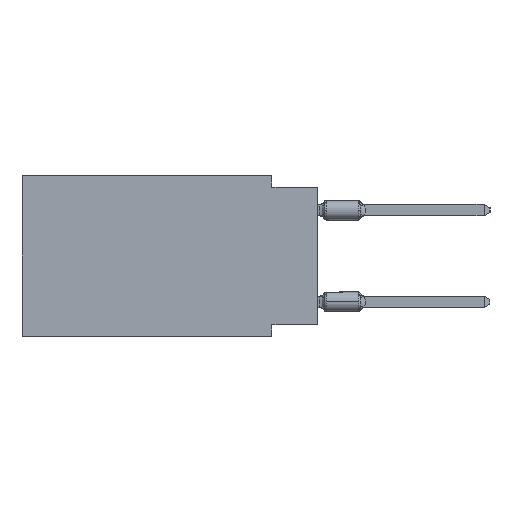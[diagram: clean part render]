
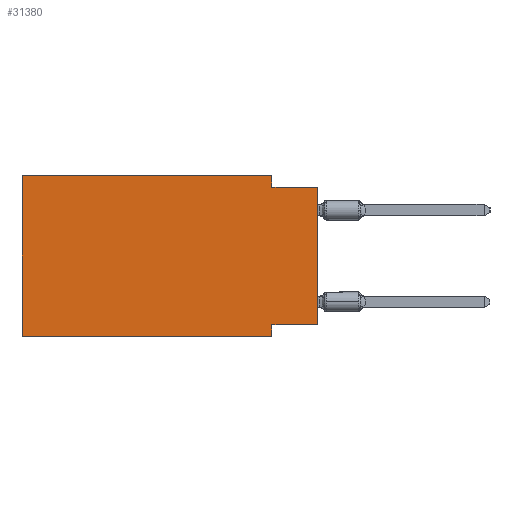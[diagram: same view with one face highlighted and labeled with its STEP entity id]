
A CAD part, left-side view. The second image highlights one B-rep face of the part: STEP entity #31380.
In plain terms, the highlighted planar face has unit normal (-1, 0, 0).
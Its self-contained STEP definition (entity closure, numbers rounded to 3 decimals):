
#2015 = EDGE_CURVE ( 'NONE', #42631, #43121, #25389, .T. ) ;
#2794 = DIRECTION ( 'NONE',  ( 0., 0., 1. ) ) ;
#2954 = VECTOR ( 'NONE', #29183, 1000. ) ;
#3737 = AXIS2_PLACEMENT_3D ( 'NONE', #24663, #42346, #38806 ) ;
#4232 = LINE ( 'NONE', #17900, #43510 ) ;
#5500 = FACE_OUTER_BOUND ( 'NONE', #38453, .T. ) ;
#5886 = ORIENTED_EDGE ( 'NONE', *, *, #20736, .F. ) ;
#5915 = CARTESIAN_POINT ( 'NONE',  ( 0., 16.383, -8.89 ) ) ;
#6879 = DIRECTION ( 'NONE',  ( 0., 0., 1. ) ) ;
#7085 = DIRECTION ( 'NONE',  ( 0., -1., 0. ) ) ;
#9016 = CARTESIAN_POINT ( 'NONE',  ( 0., 16.383, -8.89 ) ) ;
#10177 = EDGE_CURVE ( 'NONE', #32610, #34046, #17028, .T. ) ;
#10207 = CARTESIAN_POINT ( 'NONE',  ( 0., 2.54, -0.635 ) ) ;
#11324 = EDGE_CURVE ( 'NONE', #40060, #34046, #4232, .T. ) ;
#15069 = VECTOR ( 'NONE', #2794, 1000. ) ;
#16110 = EDGE_CURVE ( 'NONE', #40060, #19717, #24995, .T. ) ;
#16838 = ORIENTED_EDGE ( 'NONE', *, *, #10177, .F. ) ;
#17028 = LINE ( 'NONE', #37306, #37783 ) ;
#17112 = CARTESIAN_POINT ( 'NONE',  ( 0., 0., -0.635 ) ) ;
#17409 = VECTOR ( 'NONE', #41638, 1000. ) ;
#17900 = CARTESIAN_POINT ( 'NONE',  ( 0., 0., 0. ) ) ;
#18295 = CARTESIAN_POINT ( 'NONE',  ( 0., 0., -8.255 ) ) ;
#18673 = CARTESIAN_POINT ( 'NONE',  ( 0., 2.54, -8.89 ) ) ;
#18843 = CARTESIAN_POINT ( 'NONE',  ( 0., 0., -8.255 ) ) ;
#19096 = LINE ( 'NONE', #25693, #40429 ) ;
#19513 = EDGE_CURVE ( 'NONE', #33516, #29248, #35731, .T. ) ;
#19717 = VERTEX_POINT ( 'NONE', #30192 ) ;
#19989 = CARTESIAN_POINT ( 'NONE',  ( 0., 16.383, 0. ) ) ;
#20736 = EDGE_CURVE ( 'NONE', #19717, #29248, #19096, .T. ) ;
#20992 = VECTOR ( 'NONE', #22105, 1000. ) ;
#21790 = CARTESIAN_POINT ( 'NONE',  ( 0., 2.54, 0. ) ) ;
#22040 = ORIENTED_EDGE ( 'NONE', *, *, #2015, .F. ) ;
#22105 = DIRECTION ( 'NONE',  ( 0., -1., 0. ) ) ;
#23414 = ORIENTED_EDGE ( 'NONE', *, *, #41847, .F. ) ;
#24663 = CARTESIAN_POINT ( 'NONE',  ( 0., 16.383, 0. ) ) ;
#24995 = LINE ( 'NONE', #18843, #2954 ) ;
#25018 = ORIENTED_EDGE ( 'NONE', *, *, #39048, .F. ) ;
#25321 = DIRECTION ( 'NONE',  ( 0., -1., 0. ) ) ;
#25389 = LINE ( 'NONE', #35139, #20992 ) ;
#25693 = CARTESIAN_POINT ( 'NONE',  ( 0., 2.54, -8.89 ) ) ;
#26971 = ORIENTED_EDGE ( 'NONE', *, *, #11324, .T. ) ;
#29183 = DIRECTION ( 'NONE',  ( 0., 1., 0. ) ) ;
#29248 = VERTEX_POINT ( 'NONE', #18673 ) ;
#30192 = CARTESIAN_POINT ( 'NONE',  ( 0., 2.54, -8.255 ) ) ;
#31380 = ADVANCED_FACE ( 'NONE', ( #5500 ), #31759, .F. ) ;
#31759 = PLANE ( 'NONE',  #3737 ) ;
#32483 = ORIENTED_EDGE ( 'NONE', *, *, #16110, .F. ) ;
#32610 = VERTEX_POINT ( 'NONE', #10207 ) ;
#32993 = DIRECTION ( 'NONE',  ( 0., 0., -1. ) ) ;
#33516 = VERTEX_POINT ( 'NONE', #5915 ) ;
#34046 = VERTEX_POINT ( 'NONE', #17112 ) ;
#35139 = CARTESIAN_POINT ( 'NONE',  ( 0., 16.383, 0. ) ) ;
#35731 = LINE ( 'NONE', #9016, #37675 ) ;
#35743 = CARTESIAN_POINT ( 'NONE',  ( 0., 2.54, 0. ) ) ;
#37306 = CARTESIAN_POINT ( 'NONE',  ( 0., 0., -0.635 ) ) ;
#37675 = VECTOR ( 'NONE', #25321, 1000. ) ;
#37783 = VECTOR ( 'NONE', #7085, 1000. ) ;
#38319 = LINE ( 'NONE', #21790, #17409 ) ;
#38453 = EDGE_LOOP ( 'NONE', ( #26971, #16838, #23414, #22040, #25018, #43067, #5886, #32483 ) ) ;
#38806 = DIRECTION ( 'NONE',  ( 0., 0., -1. ) ) ;
#39048 = EDGE_CURVE ( 'NONE', #33516, #42631, #40067, .T. ) ;
#40060 = VERTEX_POINT ( 'NONE', #18295 ) ;
#40067 = LINE ( 'NONE', #19989, #15069 ) ;
#40429 = VECTOR ( 'NONE', #32993, 1000. ) ;
#40869 = CARTESIAN_POINT ( 'NONE',  ( 0., 16.383, 0. ) ) ;
#41638 = DIRECTION ( 'NONE',  ( 0., 0., -1. ) ) ;
#41847 = EDGE_CURVE ( 'NONE', #43121, #32610, #38319, .T. ) ;
#42346 = DIRECTION ( 'NONE',  ( 1., 0., 0. ) ) ;
#42631 = VERTEX_POINT ( 'NONE', #40869 ) ;
#43067 = ORIENTED_EDGE ( 'NONE', *, *, #19513, .T. ) ;
#43121 = VERTEX_POINT ( 'NONE', #35743 ) ;
#43510 = VECTOR ( 'NONE', #6879, 1000. ) ;
